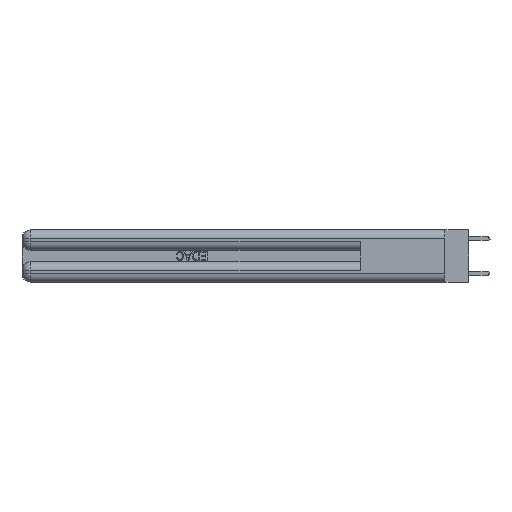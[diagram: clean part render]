
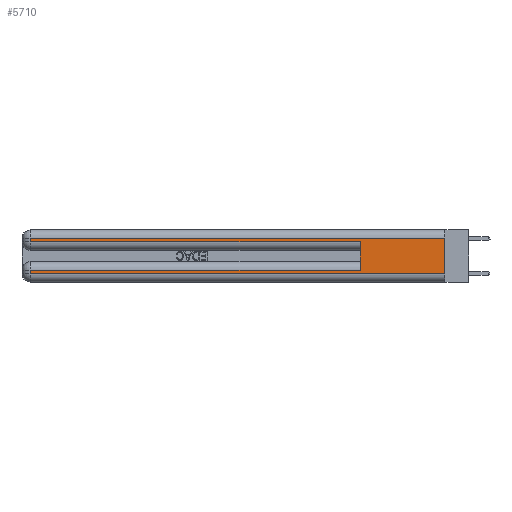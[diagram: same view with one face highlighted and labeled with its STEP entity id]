
A CAD part, left-side view. The second image highlights one B-rep face of the part: STEP entity #5710.
In plain terms, the highlighted planar face has unit normal (-1, 0, 0).
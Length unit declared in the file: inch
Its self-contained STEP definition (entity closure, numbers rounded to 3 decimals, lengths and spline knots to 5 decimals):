
#60 = DIRECTION ( 'NONE',  ( 0., -1., 0. ) ) ;
#158 = AXIS2_PLACEMENT_3D ( 'NONE', #26003, #2820, #19087 ) ;
#424 = PLANE ( 'NONE',  #158 ) ;
#602 = LINE ( 'NONE', #21070, #12285 ) ;
#838 = CARTESIAN_POINT ( 'NONE',  ( 0., 0.6, 0.145 ) ) ;
#1032 = CARTESIAN_POINT ( 'NONE',  ( 0., 2.94, 0.31 ) ) ;
#1128 = EDGE_CURVE ( 'NONE', #29436, #1137, #21292, .T. ) ;
#1137 = VERTEX_POINT ( 'NONE', #4376 ) ;
#1928 = VECTOR ( 'NONE', #15532, 39.37008 ) ;
#2232 = VECTOR ( 'NONE', #9339, 39.37008 ) ;
#2820 = DIRECTION ( 'NONE',  ( 1., 0., 0. ) ) ;
#3174 = DIRECTION ( 'NONE',  ( 0., 0., -1. ) ) ;
#3262 = CARTESIAN_POINT ( 'NONE',  ( 0., 2.94, 0.37 ) ) ;
#4376 = CARTESIAN_POINT ( 'NONE',  ( 0., 2.94, 0.285 ) ) ;
#4404 = LINE ( 'NONE', #8435, #10599 ) ;
#5271 = CARTESIAN_POINT ( 'NONE',  ( 0., 2.94, 0.06 ) ) ;
#5291 = EDGE_LOOP ( 'NONE', ( #27941, #22593, #20476, #14633, #14022, #15378, #7214, #17082 ) ) ;
#5710 = ADVANCED_FACE ( 'NONE', ( #27490 ), #424, .F. ) ;
#5731 = VERTEX_POINT ( 'NONE', #21416 ) ;
#6817 = CARTESIAN_POINT ( 'NONE',  ( 0., 0.6, 0.285 ) ) ;
#6988 = CARTESIAN_POINT ( 'NONE',  ( 0., 0., 0.37 ) ) ;
#7214 = ORIENTED_EDGE ( 'NONE', *, *, #24504, .T. ) ;
#7284 = VECTOR ( 'NONE', #12473, 39.37008 ) ;
#7459 = VECTOR ( 'NONE', #3174, 39.37008 ) ;
#8144 = LINE ( 'NONE', #29450, #1928 ) ;
#8435 = CARTESIAN_POINT ( 'NONE',  ( 0., 0., 0.085 ) ) ;
#8440 = LINE ( 'NONE', #6988, #2232 ) ;
#9339 = DIRECTION ( 'NONE',  ( 0., 0., -1. ) ) ;
#10599 = VECTOR ( 'NONE', #20014, 39.37008 ) ;
#12285 = VECTOR ( 'NONE', #60, 39.37008 ) ;
#12473 = DIRECTION ( 'NONE',  ( 0., 0., 1. ) ) ;
#13649 = LINE ( 'NONE', #3262, #7459 ) ;
#14022 = ORIENTED_EDGE ( 'NONE', *, *, #27388, .F. ) ;
#14586 = EDGE_CURVE ( 'NONE', #5731, #29436, #18304, .T. ) ;
#14633 = ORIENTED_EDGE ( 'NONE', *, *, #17954, .T. ) ;
#15378 = ORIENTED_EDGE ( 'NONE', *, *, #27017, .T. ) ;
#15532 = DIRECTION ( 'NONE',  ( 0., -1., 0. ) ) ;
#15973 = CARTESIAN_POINT ( 'NONE',  ( 0., 2.94, 0.37 ) ) ;
#16994 = CARTESIAN_POINT ( 'NONE',  ( 0., 0.6, 0.085 ) ) ;
#17082 = ORIENTED_EDGE ( 'NONE', *, *, #22594, .T. ) ;
#17194 = VERTEX_POINT ( 'NONE', #16994 ) ;
#17493 = VERTEX_POINT ( 'NONE', #6817 ) ;
#17954 = EDGE_CURVE ( 'NONE', #1137, #17493, #8144, .T. ) ;
#18304 = LINE ( 'NONE', #21881, #23738 ) ;
#18711 = VERTEX_POINT ( 'NONE', #5271 ) ;
#19087 = DIRECTION ( 'NONE',  ( 0., 0., -1. ) ) ;
#19199 = EDGE_CURVE ( 'NONE', #5731, #24932, #8440, .T. ) ;
#20014 = DIRECTION ( 'NONE',  ( 0., 1., 0. ) ) ;
#20476 = ORIENTED_EDGE ( 'NONE', *, *, #1128, .T. ) ;
#21050 = CARTESIAN_POINT ( 'NONE',  ( 0., 0., 0.06 ) ) ;
#21070 = CARTESIAN_POINT ( 'NONE',  ( 0., 0., 0.06 ) ) ;
#21292 = LINE ( 'NONE', #15973, #26742 ) ;
#21416 = CARTESIAN_POINT ( 'NONE',  ( 0., 0., 0.31 ) ) ;
#21881 = CARTESIAN_POINT ( 'NONE',  ( 0., 0., 0.31 ) ) ;
#22525 = VERTEX_POINT ( 'NONE', #25028 ) ;
#22593 = ORIENTED_EDGE ( 'NONE', *, *, #14586, .T. ) ;
#22594 = EDGE_CURVE ( 'NONE', #18711, #24932, #602, .T. ) ;
#23738 = VECTOR ( 'NONE', #28810, 39.37008 ) ;
#24504 = EDGE_CURVE ( 'NONE', #22525, #18711, #13649, .T. ) ;
#24932 = VERTEX_POINT ( 'NONE', #21050 ) ;
#25028 = CARTESIAN_POINT ( 'NONE',  ( 0., 2.94, 0.085 ) ) ;
#25841 = LINE ( 'NONE', #838, #7284 ) ;
#26003 = CARTESIAN_POINT ( 'NONE',  ( 0., 0., 0.37 ) ) ;
#26742 = VECTOR ( 'NONE', #27591, 39.37008 ) ;
#27017 = EDGE_CURVE ( 'NONE', #17194, #22525, #4404, .T. ) ;
#27388 = EDGE_CURVE ( 'NONE', #17194, #17493, #25841, .T. ) ;
#27490 = FACE_OUTER_BOUND ( 'NONE', #5291, .T. ) ;
#27591 = DIRECTION ( 'NONE',  ( 0., 0., -1. ) ) ;
#27941 = ORIENTED_EDGE ( 'NONE', *, *, #19199, .F. ) ;
#28810 = DIRECTION ( 'NONE',  ( 0., 1., 0. ) ) ;
#29436 = VERTEX_POINT ( 'NONE', #1032 ) ;
#29450 = CARTESIAN_POINT ( 'NONE',  ( 0., 0., 0.285 ) ) ;
